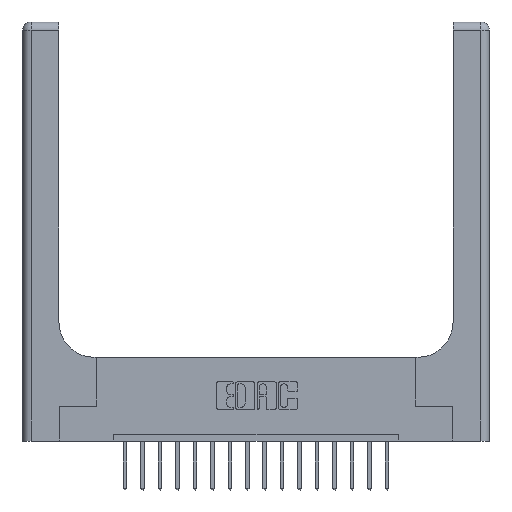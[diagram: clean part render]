
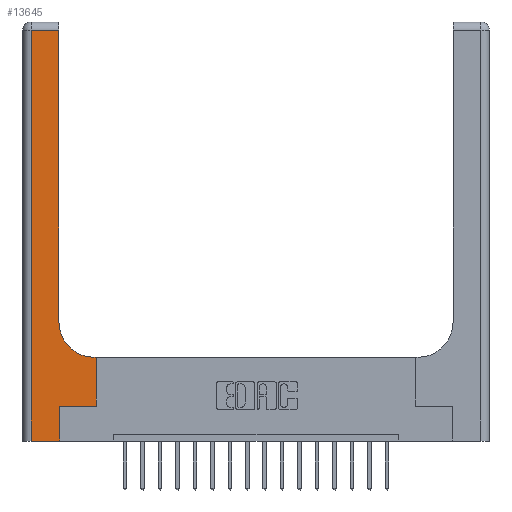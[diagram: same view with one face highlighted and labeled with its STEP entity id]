
A CAD part, top view. The second image highlights one B-rep face of the part: STEP entity #13645.
In plain terms, the highlighted planar face has unit normal (0, 0, 1).
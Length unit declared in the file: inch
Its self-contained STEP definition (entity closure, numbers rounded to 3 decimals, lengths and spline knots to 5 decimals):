
#123 = VERTEX_POINT ( 'NONE', #9248 ) ;
#132 = CARTESIAN_POINT ( 'NONE',  ( 0.26, 0.6, 0.37 ) ) ;
#314 = VERTEX_POINT ( 'NONE', #10748 ) ;
#888 = VECTOR ( 'NONE', #11338, 39.37008 ) ;
#1144 = VERTEX_POINT ( 'NONE', #3879 ) ;
#1681 = DIRECTION ( 'NONE',  ( -1., 0., 0. ) ) ;
#2161 = FACE_OUTER_BOUND ( 'NONE', #9337, .T. ) ;
#2169 = CARTESIAN_POINT ( 'NONE',  ( 0.06, 0., 0.37 ) ) ;
#2989 = ORIENTED_EDGE ( 'NONE', *, *, #9890, .T. ) ;
#3368 = LINE ( 'NONE', #15736, #888 ) ;
#3577 = DIRECTION ( 'NONE',  ( 1., 0., 0. ) ) ;
#3853 = CARTESIAN_POINT ( 'NONE',  ( 0.26, 3., 0.37 ) ) ;
#3879 = CARTESIAN_POINT ( 'NONE',  ( 0.528, 0.6, 0.37 ) ) ;
#4278 = VECTOR ( 'NONE', #10080, 39.37008 ) ;
#4387 = DIRECTION ( 'NONE',  ( 1., 0., 0. ) ) ;
#4425 = DIRECTION ( 'NONE',  ( -1., 0., 0. ) ) ;
#4703 = CARTESIAN_POINT ( 'NONE',  ( 0., 2.94, 0.37 ) ) ;
#4772 = VERTEX_POINT ( 'NONE', #11397 ) ;
#4871 = LINE ( 'NONE', #3853, #7109 ) ;
#4885 = VECTOR ( 'NONE', #14495, 39.37008 ) ;
#5295 = AXIS2_PLACEMENT_3D ( 'NONE', #13169, #15810, #4425 ) ;
#5506 = VECTOR ( 'NONE', #13264, 39.37008 ) ;
#5535 = VERTEX_POINT ( 'NONE', #2169 ) ;
#6621 = ORIENTED_EDGE ( 'NONE', *, *, #9991, .T. ) ;
#6751 = ORIENTED_EDGE ( 'NONE', *, *, #17641, .T. ) ;
#7109 = VECTOR ( 'NONE', #15716, 39.37008 ) ;
#7283 = CARTESIAN_POINT ( 'NONE',  ( 0., 0., 0.37 ) ) ;
#7393 = CIRCLE ( 'NONE', #10707, 0.25 ) ;
#7521 = EDGE_CURVE ( 'NONE', #8599, #8135, #7393, .T. ) ;
#8001 = EDGE_CURVE ( 'NONE', #5535, #13975, #18200, .T. ) ;
#8135 = VERTEX_POINT ( 'NONE', #10394 ) ;
#8599 = VERTEX_POINT ( 'NONE', #10393 ) ;
#8696 = PLANE ( 'NONE',  #5295 ) ;
#8867 = EDGE_CURVE ( 'NONE', #13975, #4772, #3368, .T. ) ;
#9248 = CARTESIAN_POINT ( 'NONE',  ( 0.26, 2.94, 0.37 ) ) ;
#9337 = EDGE_LOOP ( 'NONE', ( #2989, #6751, #15705, #18239, #14054, #11677, #6621, #13131, #16432 ) ) ;
#9806 = CARTESIAN_POINT ( 'NONE',  ( 0.265, 0., 0.37 ) ) ;
#9845 = LINE ( 'NONE', #11612, #10758 ) ;
#9890 = EDGE_CURVE ( 'NONE', #8135, #123, #4871, .T. ) ;
#9991 = EDGE_CURVE ( 'NONE', #10595, #1144, #9845, .T. ) ;
#10080 = DIRECTION ( 'NONE',  ( 1., 0., 0. ) ) ;
#10310 = CARTESIAN_POINT ( 'NONE',  ( 0.06, 3., 0.37 ) ) ;
#10393 = CARTESIAN_POINT ( 'NONE',  ( 0.51, 0.6, 0.37 ) ) ;
#10394 = CARTESIAN_POINT ( 'NONE',  ( 0.26, 0.85, 0.37 ) ) ;
#10512 = LINE ( 'NONE', #4703, #16780 ) ;
#10595 = VERTEX_POINT ( 'NONE', #11737 ) ;
#10707 = AXIS2_PLACEMENT_3D ( 'NONE', #16491, #12166, #3577 ) ;
#10748 = CARTESIAN_POINT ( 'NONE',  ( 0.06, 2.94, 0.37 ) ) ;
#10758 = VECTOR ( 'NONE', #14517, 39.37008 ) ;
#11338 = DIRECTION ( 'NONE',  ( 0., 1., 0. ) ) ;
#11384 = EDGE_CURVE ( 'NONE', #1144, #8599, #14808, .T. ) ;
#11397 = CARTESIAN_POINT ( 'NONE',  ( 0.265, 0.25, 0.37 ) ) ;
#11612 = CARTESIAN_POINT ( 'NONE',  ( 0.528, 0.25, 0.37 ) ) ;
#11677 = ORIENTED_EDGE ( 'NONE', *, *, #18472, .T. ) ;
#11737 = CARTESIAN_POINT ( 'NONE',  ( 0.528, 0.25, 0.37 ) ) ;
#12040 = LINE ( 'NONE', #13089, #18102 ) ;
#12166 = DIRECTION ( 'NONE',  ( 0., 0., -1. ) ) ;
#13089 = CARTESIAN_POINT ( 'NONE',  ( 0.265, 0.25, 0.37 ) ) ;
#13131 = ORIENTED_EDGE ( 'NONE', *, *, #11384, .T. ) ;
#13169 = CARTESIAN_POINT ( 'NONE',  ( 0., 3., 0.37 ) ) ;
#13264 = DIRECTION ( 'NONE',  ( 0., -1., 0. ) ) ;
#13645 = ADVANCED_FACE ( 'NONE', ( #2161 ), #8696, .F. ) ;
#13975 = VERTEX_POINT ( 'NONE', #9806 ) ;
#14054 = ORIENTED_EDGE ( 'NONE', *, *, #8867, .T. ) ;
#14495 = DIRECTION ( 'NONE',  ( -1., 0., 0. ) ) ;
#14517 = DIRECTION ( 'NONE',  ( 0., 1., 0. ) ) ;
#14808 = LINE ( 'NONE', #132, #4885 ) ;
#15431 = LINE ( 'NONE', #10310, #5506 ) ;
#15705 = ORIENTED_EDGE ( 'NONE', *, *, #18649, .T. ) ;
#15716 = DIRECTION ( 'NONE',  ( 0., 1., 0. ) ) ;
#15736 = CARTESIAN_POINT ( 'NONE',  ( 0.265, 0., 0.37 ) ) ;
#15810 = DIRECTION ( 'NONE',  ( 0., 0., -1. ) ) ;
#16432 = ORIENTED_EDGE ( 'NONE', *, *, #7521, .T. ) ;
#16491 = CARTESIAN_POINT ( 'NONE',  ( 0.51, 0.85, 0.37 ) ) ;
#16780 = VECTOR ( 'NONE', #1681, 39.37008 ) ;
#17641 = EDGE_CURVE ( 'NONE', #123, #314, #10512, .T. ) ;
#18102 = VECTOR ( 'NONE', #4387, 39.37008 ) ;
#18200 = LINE ( 'NONE', #7283, #4278 ) ;
#18239 = ORIENTED_EDGE ( 'NONE', *, *, #8001, .T. ) ;
#18472 = EDGE_CURVE ( 'NONE', #4772, #10595, #12040, .T. ) ;
#18649 = EDGE_CURVE ( 'NONE', #314, #5535, #15431, .T. ) ;
